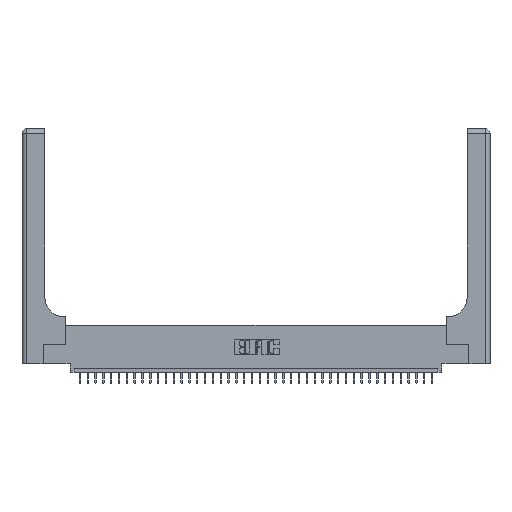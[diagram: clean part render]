
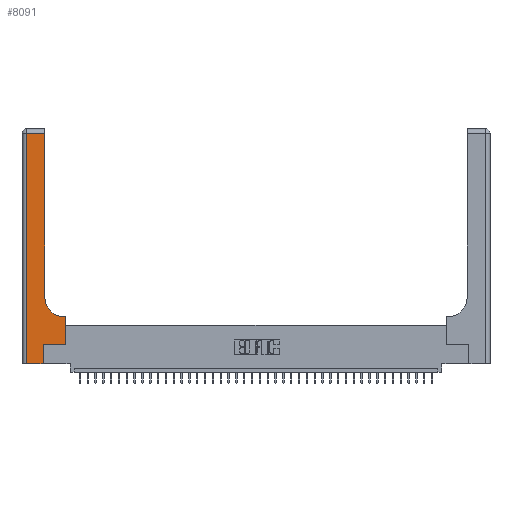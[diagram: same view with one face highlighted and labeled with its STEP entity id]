
A CAD part, top view. The second image highlights one B-rep face of the part: STEP entity #8091.
In plain terms, the highlighted planar face has unit normal (0, 0, 1).
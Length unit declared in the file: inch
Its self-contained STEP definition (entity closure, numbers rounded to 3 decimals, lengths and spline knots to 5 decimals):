
#3 = VERTEX_POINT ( 'NONE', #13481 ) ;
#734 = VECTOR ( 'NONE', #4090, 39.37008 ) ;
#1008 = DIRECTION ( 'NONE',  ( 0., 0., -1. ) ) ;
#1907 = CARTESIAN_POINT ( 'NONE',  ( 0., 2.94, 0.37 ) ) ;
#2479 = ORIENTED_EDGE ( 'NONE', *, *, #38840, .T. ) ;
#2718 = AXIS2_PLACEMENT_3D ( 'NONE', #6628, #1008, #18989 ) ;
#2870 = CARTESIAN_POINT ( 'NONE',  ( 0.269, 0.25, 0.37 ) ) ;
#3246 = EDGE_CURVE ( 'NONE', #22910, #33278, #39327, .T. ) ;
#3498 = LINE ( 'NONE', #30860, #734 ) ;
#3523 = EDGE_LOOP ( 'NONE', ( #4558, #2479, #19437, #15901, #14061, #11057, #14474, #36727, #10964 ) ) ;
#4090 = DIRECTION ( 'NONE',  ( 0., -1., 0. ) ) ;
#4558 = ORIENTED_EDGE ( 'NONE', *, *, #19642, .T. ) ;
#4980 = CARTESIAN_POINT ( 'NONE',  ( 0.2915, 0.6, 0.37 ) ) ;
#5298 = CARTESIAN_POINT ( 'NONE',  ( 0., 0., 0.37 ) ) ;
#5669 = VECTOR ( 'NONE', #13458, 39.37008 ) ;
#6628 = CARTESIAN_POINT ( 'NONE',  ( 0., 3., 0.37 ) ) ;
#8091 = ADVANCED_FACE ( 'NONE', ( #24789 ), #27982, .F. ) ;
#8112 = EDGE_CURVE ( 'NONE', #10095, #30839, #31170, .T. ) ;
#8305 = LINE ( 'NONE', #1907, #14260 ) ;
#8531 = DIRECTION ( 'NONE',  ( 0., 1., 0. ) ) ;
#8655 = EDGE_CURVE ( 'NONE', #3, #18410, #3498, .T. ) ;
#8914 = CARTESIAN_POINT ( 'NONE',  ( 0.5585, 0.25, 0.37 ) ) ;
#10095 = VERTEX_POINT ( 'NONE', #2870 ) ;
#10895 = DIRECTION ( 'NONE',  ( -1., 0., 0. ) ) ;
#10964 = ORIENTED_EDGE ( 'NONE', *, *, #15742, .T. ) ;
#11057 = ORIENTED_EDGE ( 'NONE', *, *, #8112, .T. ) ;
#11643 = VECTOR ( 'NONE', #14557, 39.37008 ) ;
#11904 = DIRECTION ( 'NONE',  ( 0., 0., -1. ) ) ;
#12297 = DIRECTION ( 'NONE',  ( 0., 1., 0. ) ) ;
#12571 = CIRCLE ( 'NONE', #34870, 0.25 ) ;
#13458 = DIRECTION ( 'NONE',  ( 0., 1., 0. ) ) ;
#13481 = CARTESIAN_POINT ( 'NONE',  ( 0.06, 2.94, 0.37 ) ) ;
#14061 = ORIENTED_EDGE ( 'NONE', *, *, #33716, .T. ) ;
#14260 = VECTOR ( 'NONE', #10895, 39.37008 ) ;
#14315 = CARTESIAN_POINT ( 'NONE',  ( 0.269, 0., 0.37 ) ) ;
#14474 = ORIENTED_EDGE ( 'NONE', *, *, #19584, .T. ) ;
#14557 = DIRECTION ( 'NONE',  ( -1., 0., 0. ) ) ;
#14698 = CARTESIAN_POINT ( 'NONE',  ( 0.06, 0., 0.37 ) ) ;
#14720 = LINE ( 'NONE', #14315, #31893 ) ;
#15742 = EDGE_CURVE ( 'NONE', #33278, #38842, #12571, .T. ) ;
#15901 = ORIENTED_EDGE ( 'NONE', *, *, #20819, .T. ) ;
#16000 = CARTESIAN_POINT ( 'NONE',  ( 0.269, 0.25, 0.37 ) ) ;
#16243 = VERTEX_POINT ( 'NONE', #23378 ) ;
#18410 = VERTEX_POINT ( 'NONE', #14698 ) ;
#18989 = DIRECTION ( 'NONE',  ( -1., 0., 0. ) ) ;
#19437 = ORIENTED_EDGE ( 'NONE', *, *, #8655, .T. ) ;
#19584 = EDGE_CURVE ( 'NONE', #30839, #22910, #24094, .T. ) ;
#19642 = EDGE_CURVE ( 'NONE', #38842, #31470, #25076, .T. ) ;
#20471 = CARTESIAN_POINT ( 'NONE',  ( 0.2915, 0.85, 0.37 ) ) ;
#20819 = EDGE_CURVE ( 'NONE', #18410, #16243, #23464, .T. ) ;
#21089 = DIRECTION ( 'NONE',  ( 1., 0., 0. ) ) ;
#22910 = VERTEX_POINT ( 'NONE', #30123 ) ;
#23378 = CARTESIAN_POINT ( 'NONE',  ( 0.269, 0., 0.37 ) ) ;
#23464 = LINE ( 'NONE', #5298, #24888 ) ;
#24094 = LINE ( 'NONE', #8914, #36905 ) ;
#24789 = FACE_OUTER_BOUND ( 'NONE', #3523, .T. ) ;
#24888 = VECTOR ( 'NONE', #35626, 39.37008 ) ;
#25076 = LINE ( 'NONE', #37829, #5669 ) ;
#25602 = CARTESIAN_POINT ( 'NONE',  ( 0.5415, 0.6, 0.37 ) ) ;
#27982 = PLANE ( 'NONE',  #2718 ) ;
#30123 = CARTESIAN_POINT ( 'NONE',  ( 0.5585, 0.6, 0.37 ) ) ;
#30839 = VERTEX_POINT ( 'NONE', #34814 ) ;
#30860 = CARTESIAN_POINT ( 'NONE',  ( 0.06, 3., 0.37 ) ) ;
#31170 = LINE ( 'NONE', #16000, #32686 ) ;
#31470 = VERTEX_POINT ( 'NONE', #38770 ) ;
#31893 = VECTOR ( 'NONE', #8531, 39.37008 ) ;
#32686 = VECTOR ( 'NONE', #37558, 39.37008 ) ;
#33278 = VERTEX_POINT ( 'NONE', #25602 ) ;
#33716 = EDGE_CURVE ( 'NONE', #16243, #10095, #14720, .T. ) ;
#34814 = CARTESIAN_POINT ( 'NONE',  ( 0.5585, 0.25, 0.37 ) ) ;
#34870 = AXIS2_PLACEMENT_3D ( 'NONE', #39458, #11904, #21089 ) ;
#35626 = DIRECTION ( 'NONE',  ( 1., 0., 0. ) ) ;
#36727 = ORIENTED_EDGE ( 'NONE', *, *, #3246, .T. ) ;
#36905 = VECTOR ( 'NONE', #12297, 39.37008 ) ;
#37558 = DIRECTION ( 'NONE',  ( 1., 0., 0. ) ) ;
#37829 = CARTESIAN_POINT ( 'NONE',  ( 0.2915, 3., 0.37 ) ) ;
#38770 = CARTESIAN_POINT ( 'NONE',  ( 0.2915, 2.94, 0.37 ) ) ;
#38840 = EDGE_CURVE ( 'NONE', #31470, #3, #8305, .T. ) ;
#38842 = VERTEX_POINT ( 'NONE', #20471 ) ;
#39327 = LINE ( 'NONE', #4980, #11643 ) ;
#39458 = CARTESIAN_POINT ( 'NONE',  ( 0.5415, 0.85, 0.37 ) ) ;
